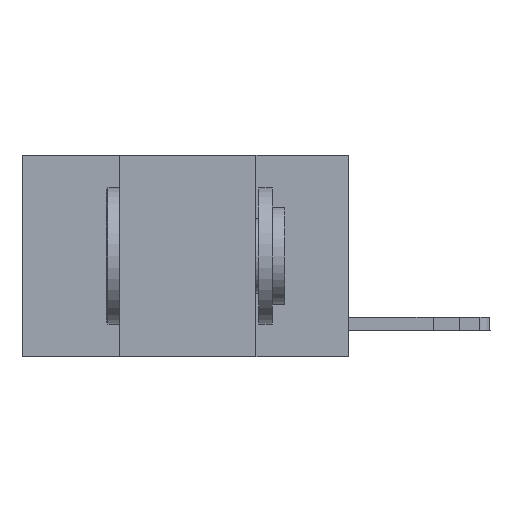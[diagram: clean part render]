
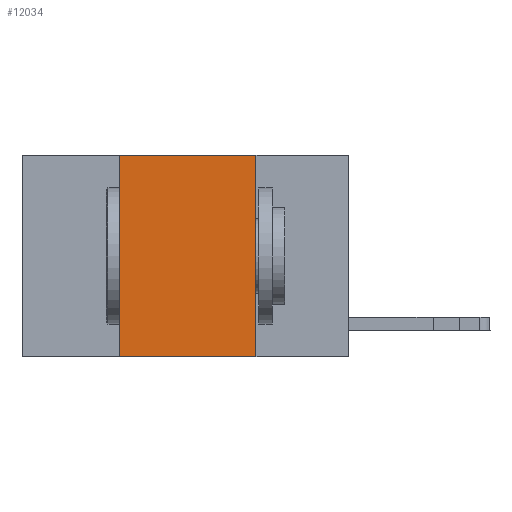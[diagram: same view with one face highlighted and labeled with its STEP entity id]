
A CAD part, left-side view. The second image highlights one B-rep face of the part: STEP entity #12034.
In plain terms, the highlighted planar face has unit normal (-1, 0, 0).
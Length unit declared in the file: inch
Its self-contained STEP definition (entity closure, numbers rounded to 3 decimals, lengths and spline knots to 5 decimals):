
#387 = EDGE_CURVE ( 'NONE', #9477, #3592, #3962, .T. ) ;
#629 = VECTOR ( 'NONE', #7186, 39.37008 ) ;
#3167 = VECTOR ( 'NONE', #8445, 39.37008 ) ;
#3320 = VERTEX_POINT ( 'NONE', #8032 ) ;
#3592 = VERTEX_POINT ( 'NONE', #6587 ) ;
#3886 = ORIENTED_EDGE ( 'NONE', *, *, #11677, .F. ) ;
#3962 = LINE ( 'NONE', #7180, #629 ) ;
#4720 = PLANE ( 'NONE',  #7315 ) ;
#5675 = DIRECTION ( 'NONE',  ( 0., -1., 0. ) ) ;
#6246 = VECTOR ( 'NONE', #8765, 39.37008 ) ;
#6566 = CARTESIAN_POINT ( 'NONE',  ( 0., 0.17, 0. ) ) ;
#6587 = CARTESIAN_POINT ( 'NONE',  ( 0., 0.42, 0. ) ) ;
#7014 = DIRECTION ( 'NONE',  ( 1., 0., 0. ) ) ;
#7180 = CARTESIAN_POINT ( 'NONE',  ( 0., 0.42, 0. ) ) ;
#7186 = DIRECTION ( 'NONE',  ( 0., 0., 1. ) ) ;
#7315 = AXIS2_PLACEMENT_3D ( 'NONE', #13472, #7014, #14463 ) ;
#8032 = CARTESIAN_POINT ( 'NONE',  ( 0., 0.17, -0.37 ) ) ;
#8338 = CARTESIAN_POINT ( 'NONE',  ( 0., 0.17, 0. ) ) ;
#8445 = DIRECTION ( 'NONE',  ( 0., -1., 0. ) ) ;
#8642 = FACE_OUTER_BOUND ( 'NONE', #10486, .T. ) ;
#8765 = DIRECTION ( 'NONE',  ( 0., 0., -1. ) ) ;
#8939 = CARTESIAN_POINT ( 'NONE',  ( 0., 0.42, -0.37 ) ) ;
#8955 = LINE ( 'NONE', #9574, #3167 ) ;
#9477 = VERTEX_POINT ( 'NONE', #8939 ) ;
#9574 = CARTESIAN_POINT ( 'NONE',  ( 0., 0.6, 0. ) ) ;
#10053 = CARTESIAN_POINT ( 'NONE',  ( 0., 0.6, -0.37 ) ) ;
#10081 = LINE ( 'NONE', #10053, #12601 ) ;
#10486 = EDGE_LOOP ( 'NONE', ( #3886, #12424, #12502, #12688 ) ) ;
#11360 = VERTEX_POINT ( 'NONE', #8338 ) ;
#11677 = EDGE_CURVE ( 'NONE', #11360, #3320, #12684, .T. ) ;
#12034 = ADVANCED_FACE ( 'NONE', ( #8642 ), #4720, .F. ) ;
#12424 = ORIENTED_EDGE ( 'NONE', *, *, #13141, .F. ) ;
#12502 = ORIENTED_EDGE ( 'NONE', *, *, #387, .F. ) ;
#12601 = VECTOR ( 'NONE', #5675, 39.37008 ) ;
#12684 = LINE ( 'NONE', #6566, #6246 ) ;
#12688 = ORIENTED_EDGE ( 'NONE', *, *, #13461, .T. ) ;
#13141 = EDGE_CURVE ( 'NONE', #3592, #11360, #8955, .T. ) ;
#13461 = EDGE_CURVE ( 'NONE', #9477, #3320, #10081, .T. ) ;
#13472 = CARTESIAN_POINT ( 'NONE',  ( 0., 0.6, 0. ) ) ;
#14463 = DIRECTION ( 'NONE',  ( 0., 0., -1. ) ) ;
